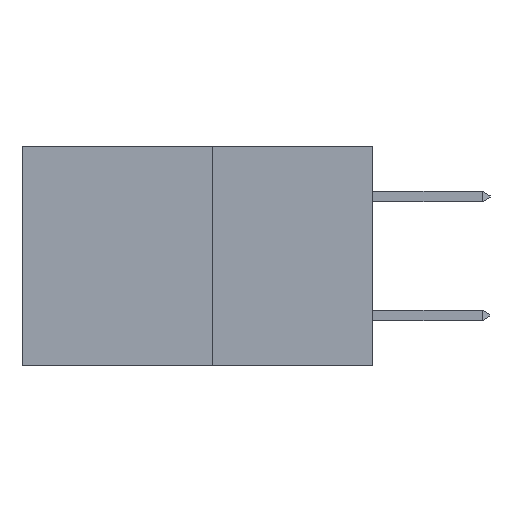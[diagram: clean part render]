
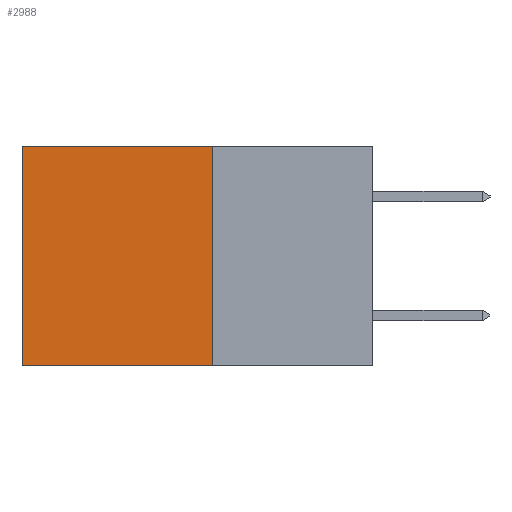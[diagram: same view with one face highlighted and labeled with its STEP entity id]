
A CAD part, left-side view. The second image highlights one B-rep face of the part: STEP entity #2988.
In plain terms, the highlighted planar face has unit normal (-1, 0, 0).
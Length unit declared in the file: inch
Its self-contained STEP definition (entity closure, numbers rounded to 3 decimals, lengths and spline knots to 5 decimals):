
#783 = FACE_OUTER_BOUND ( 'NONE', #12270, .T. ) ;
#1631 = DIRECTION ( 'NONE',  ( 0., 0., -1. ) ) ;
#2988 = ADVANCED_FACE ( 'NONE', ( #783 ), #29656, .F. ) ;
#3389 = VERTEX_POINT ( 'NONE', #16959 ) ;
#3912 = CARTESIAN_POINT ( 'NONE',  ( 0.277, 0.27, -0.37 ) ) ;
#5520 = EDGE_CURVE ( 'NONE', #28009, #19693, #9571, .T. ) ;
#6928 = VERTEX_POINT ( 'NONE', #7832 ) ;
#7525 = VECTOR ( 'NONE', #13395, 39.37008 ) ;
#7832 = CARTESIAN_POINT ( 'NONE',  ( 0.277, 0.59, 0. ) ) ;
#9092 = ORIENTED_EDGE ( 'NONE', *, *, #22839, .T. ) ;
#9571 = LINE ( 'NONE', #14684, #14303 ) ;
#10221 = ORIENTED_EDGE ( 'NONE', *, *, #28828, .F. ) ;
#12270 = EDGE_LOOP ( 'NONE', ( #22491, #10221, #29972, #9092 ) ) ;
#13096 = CARTESIAN_POINT ( 'NONE',  ( 0.277, 0.27, 0. ) ) ;
#13395 = DIRECTION ( 'NONE',  ( 0., 1., 0. ) ) ;
#14303 = VECTOR ( 'NONE', #21809, 39.37008 ) ;
#14456 = LINE ( 'NONE', #29751, #7525 ) ;
#14649 = CARTESIAN_POINT ( 'NONE',  ( 0.277, 0.59, -0.37 ) ) ;
#14684 = CARTESIAN_POINT ( 'NONE',  ( 0.277, 0.27, -0.37 ) ) ;
#15645 = DIRECTION ( 'NONE',  ( 1., 0., 0. ) ) ;
#16495 = VECTOR ( 'NONE', #25689, 39.37008 ) ;
#16959 = CARTESIAN_POINT ( 'NONE',  ( 0.277, 0.59, -0.37 ) ) ;
#17025 = DIRECTION ( 'NONE',  ( 0., 0., -1. ) ) ;
#19693 = VERTEX_POINT ( 'NONE', #27920 ) ;
#21809 = DIRECTION ( 'NONE',  ( 0., 0., -1. ) ) ;
#22491 = ORIENTED_EDGE ( 'NONE', *, *, #23737, .T. ) ;
#22839 = EDGE_CURVE ( 'NONE', #28009, #6928, #28931, .T. ) ;
#23362 = CARTESIAN_POINT ( 'NONE',  ( 0.277, 0.27, 0. ) ) ;
#23737 = EDGE_CURVE ( 'NONE', #6928, #3389, #28143, .T. ) ;
#25689 = DIRECTION ( 'NONE',  ( 0., 1., 0. ) ) ;
#27920 = CARTESIAN_POINT ( 'NONE',  ( 0.277, 0.27, -0.37 ) ) ;
#28009 = VERTEX_POINT ( 'NONE', #13096 ) ;
#28143 = LINE ( 'NONE', #14649, #28865 ) ;
#28552 = AXIS2_PLACEMENT_3D ( 'NONE', #3912, #15645, #1631 ) ;
#28828 = EDGE_CURVE ( 'NONE', #19693, #3389, #14456, .T. ) ;
#28865 = VECTOR ( 'NONE', #17025, 39.37008 ) ;
#28931 = LINE ( 'NONE', #23362, #16495 ) ;
#29656 = PLANE ( 'NONE',  #28552 ) ;
#29751 = CARTESIAN_POINT ( 'NONE',  ( 0.277, 0.27, -0.37 ) ) ;
#29972 = ORIENTED_EDGE ( 'NONE', *, *, #5520, .F. ) ;
